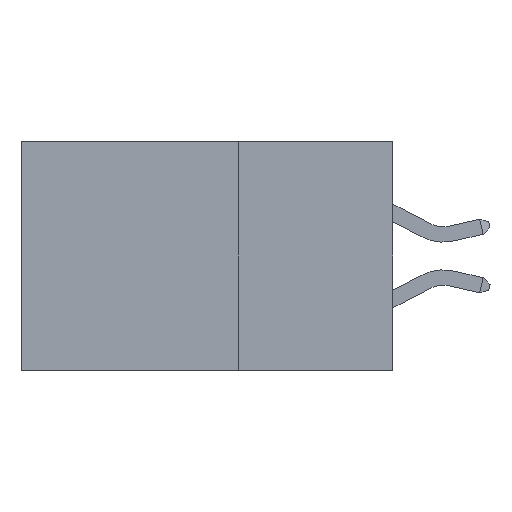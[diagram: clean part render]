
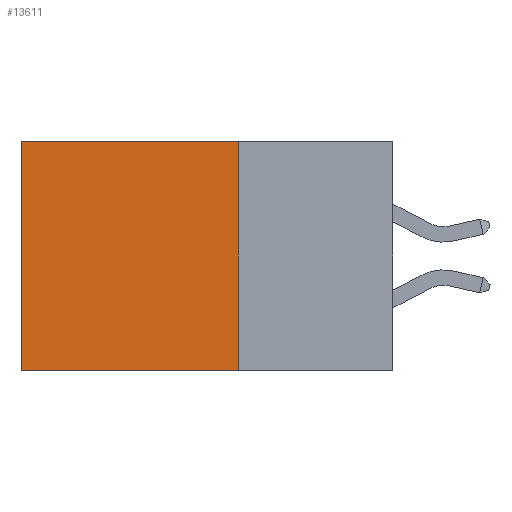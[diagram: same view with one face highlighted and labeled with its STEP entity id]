
A CAD part, left-side view. The second image highlights one B-rep face of the part: STEP entity #13611.
In plain terms, the highlighted planar face has unit normal (-1, 0, 0).
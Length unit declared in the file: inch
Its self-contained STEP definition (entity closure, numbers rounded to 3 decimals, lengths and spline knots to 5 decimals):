
#582 = LINE ( 'NONE', #21208, #10364 ) ;
#935 = CARTESIAN_POINT ( 'NONE',  ( 0.2875, 0.25, -0.37 ) ) ;
#1993 = EDGE_CURVE ( 'NONE', #7248, #5616, #24386, .T. ) ;
#2402 = ORIENTED_EDGE ( 'NONE', *, *, #2869, .T. ) ;
#2742 = EDGE_CURVE ( 'NONE', #3061, #12004, #9449, .T. ) ;
#2869 = EDGE_CURVE ( 'NONE', #12004, #5616, #582, .T. ) ;
#3061 = VERTEX_POINT ( 'NONE', #12040 ) ;
#3065 = VECTOR ( 'NONE', #16650, 39.37008 ) ;
#5616 = VERTEX_POINT ( 'NONE', #14649 ) ;
#7248 = VERTEX_POINT ( 'NONE', #935 ) ;
#9449 = LINE ( 'NONE', #12617, #3065 ) ;
#9533 = ORIENTED_EDGE ( 'NONE', *, *, #1993, .F. ) ;
#10364 = VECTOR ( 'NONE', #13668, 39.37008 ) ;
#10854 = LINE ( 'NONE', #21504, #20700 ) ;
#11384 = ORIENTED_EDGE ( 'NONE', *, *, #2742, .T. ) ;
#11439 = VECTOR ( 'NONE', #19337, 39.37008 ) ;
#12004 = VERTEX_POINT ( 'NONE', #23556 ) ;
#12040 = CARTESIAN_POINT ( 'NONE',  ( 0.2875, 0.25, 0. ) ) ;
#12617 = CARTESIAN_POINT ( 'NONE',  ( 0.2875, 0.25, 0. ) ) ;
#13611 = ADVANCED_FACE ( 'NONE', ( #18329 ), #21614, .F. ) ;
#13668 = DIRECTION ( 'NONE',  ( 0., 0., -1. ) ) ;
#14649 = CARTESIAN_POINT ( 'NONE',  ( 0.2875, 0.6, -0.37 ) ) ;
#15395 = EDGE_CURVE ( 'NONE', #3061, #7248, #10854, .T. ) ;
#16650 = DIRECTION ( 'NONE',  ( 0., 1., 0. ) ) ;
#18329 = FACE_OUTER_BOUND ( 'NONE', #22810, .T. ) ;
#18790 = AXIS2_PLACEMENT_3D ( 'NONE', #19908, #19651, #23691 ) ;
#19337 = DIRECTION ( 'NONE',  ( 0., 1., 0. ) ) ;
#19651 = DIRECTION ( 'NONE',  ( 1., 0., 0. ) ) ;
#19908 = CARTESIAN_POINT ( 'NONE',  ( 0.2875, 0.25, 0. ) ) ;
#20601 = ORIENTED_EDGE ( 'NONE', *, *, #15395, .F. ) ;
#20700 = VECTOR ( 'NONE', #23492, 39.37008 ) ;
#21208 = CARTESIAN_POINT ( 'NONE',  ( 0.2875, 0.6, 0. ) ) ;
#21388 = CARTESIAN_POINT ( 'NONE',  ( 0.2875, 0.25, -0.37 ) ) ;
#21504 = CARTESIAN_POINT ( 'NONE',  ( 0.2875, 0.25, 0. ) ) ;
#21614 = PLANE ( 'NONE',  #18790 ) ;
#22810 = EDGE_LOOP ( 'NONE', ( #2402, #9533, #20601, #11384 ) ) ;
#23492 = DIRECTION ( 'NONE',  ( 0., 0., -1. ) ) ;
#23556 = CARTESIAN_POINT ( 'NONE',  ( 0.2875, 0.6, 0. ) ) ;
#23691 = DIRECTION ( 'NONE',  ( 0., 0., -1. ) ) ;
#24386 = LINE ( 'NONE', #21388, #11439 ) ;
